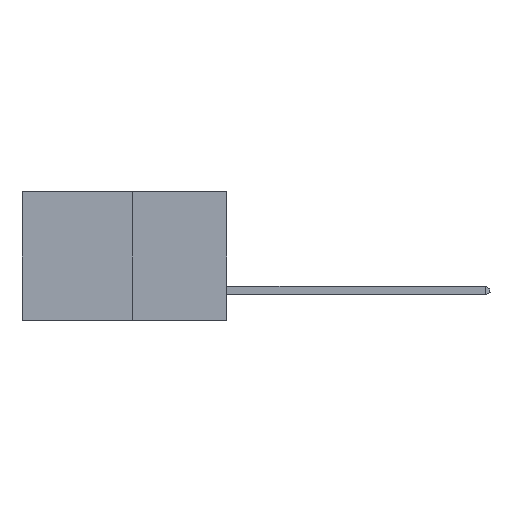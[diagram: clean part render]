
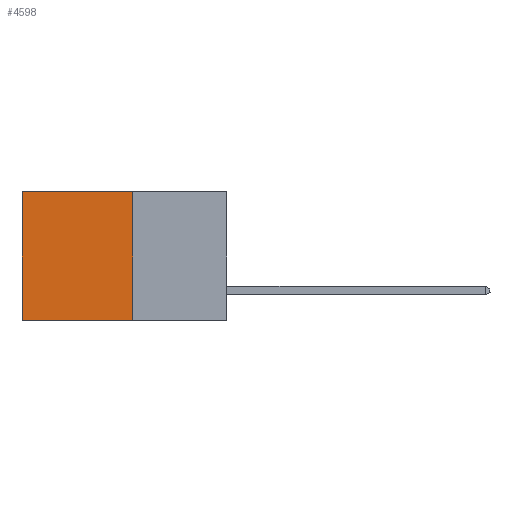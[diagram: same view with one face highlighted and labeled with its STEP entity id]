
A CAD part, left-side view. The second image highlights one B-rep face of the part: STEP entity #4598.
In plain terms, the highlighted planar face has unit normal (-1, 0, 0).
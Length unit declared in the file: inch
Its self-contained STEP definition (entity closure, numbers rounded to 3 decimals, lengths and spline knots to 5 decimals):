
#93 = EDGE_CURVE ( 'NONE', #13577, #10912, #18461, .T. ) ;
#1243 = CARTESIAN_POINT ( 'NONE',  ( 0.277, 0.27, 0. ) ) ;
#1268 = ORIENTED_EDGE ( 'NONE', *, *, #2522, .T. ) ;
#1854 = DIRECTION ( 'NONE',  ( 0., 1., 0. ) ) ;
#2522 = EDGE_CURVE ( 'NONE', #20521, #4796, #14523, .T. ) ;
#4576 = ORIENTED_EDGE ( 'NONE', *, *, #4648, .T. ) ;
#4598 = ADVANCED_FACE ( 'NONE', ( #12438 ), #6135, .F. ) ;
#4648 = EDGE_CURVE ( 'NONE', #4796, #10912, #19911, .T. ) ;
#4796 = VERTEX_POINT ( 'NONE', #8901 ) ;
#5560 = DIRECTION ( 'NONE',  ( 1., 0., 0. ) ) ;
#6135 = PLANE ( 'NONE',  #19987 ) ;
#7971 = EDGE_LOOP ( 'NONE', ( #4576, #20000, #11321, #1268 ) ) ;
#8901 = CARTESIAN_POINT ( 'NONE',  ( 0.277, 0.59, 0. ) ) ;
#9145 = CARTESIAN_POINT ( 'NONE',  ( 0.277, 0.27, -0.37 ) ) ;
#10113 = LINE ( 'NONE', #9145, #18056 ) ;
#10716 = DIRECTION ( 'NONE',  ( 0., 0., -1. ) ) ;
#10912 = VERTEX_POINT ( 'NONE', #16604 ) ;
#11182 = CARTESIAN_POINT ( 'NONE',  ( 0.277, 0.27, 0. ) ) ;
#11321 = ORIENTED_EDGE ( 'NONE', *, *, #16574, .F. ) ;
#11969 = VECTOR ( 'NONE', #16810, 39.37008 ) ;
#12438 = FACE_OUTER_BOUND ( 'NONE', #7971, .T. ) ;
#12882 = DIRECTION ( 'NONE',  ( 0., 0., -1. ) ) ;
#13577 = VERTEX_POINT ( 'NONE', #18493 ) ;
#14182 = VECTOR ( 'NONE', #15620, 39.37008 ) ;
#14523 = LINE ( 'NONE', #11182, #18295 ) ;
#15620 = DIRECTION ( 'NONE',  ( 0., 1., 0. ) ) ;
#16111 = CARTESIAN_POINT ( 'NONE',  ( 0.277, 0.59, -0.37 ) ) ;
#16574 = EDGE_CURVE ( 'NONE', #20521, #13577, #10113, .T. ) ;
#16604 = CARTESIAN_POINT ( 'NONE',  ( 0.277, 0.59, -0.37 ) ) ;
#16810 = DIRECTION ( 'NONE',  ( 0., 0., -1. ) ) ;
#17359 = CARTESIAN_POINT ( 'NONE',  ( 0.277, 0.27, -0.37 ) ) ;
#18056 = VECTOR ( 'NONE', #10716, 39.37008 ) ;
#18295 = VECTOR ( 'NONE', #1854, 39.37008 ) ;
#18461 = LINE ( 'NONE', #18721, #14182 ) ;
#18493 = CARTESIAN_POINT ( 'NONE',  ( 0.277, 0.27, -0.37 ) ) ;
#18721 = CARTESIAN_POINT ( 'NONE',  ( 0.277, 0.27, -0.37 ) ) ;
#19911 = LINE ( 'NONE', #16111, #11969 ) ;
#19987 = AXIS2_PLACEMENT_3D ( 'NONE', #17359, #5560, #12882 ) ;
#20000 = ORIENTED_EDGE ( 'NONE', *, *, #93, .F. ) ;
#20521 = VERTEX_POINT ( 'NONE', #1243 ) ;
